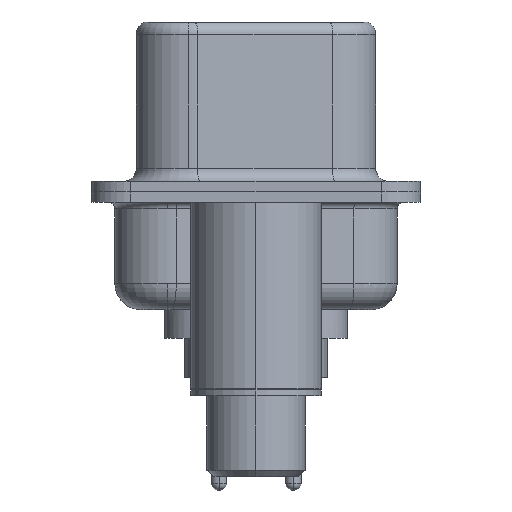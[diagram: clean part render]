
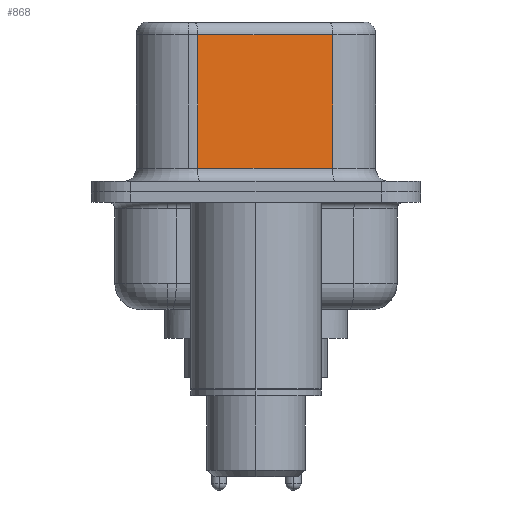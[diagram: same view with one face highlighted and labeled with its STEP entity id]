
A CAD part, left-side view. The second image highlights one B-rep face of the part: STEP entity #868.
In plain terms, the highlighted planar face has unit normal (-0.985, -0.174, 0).
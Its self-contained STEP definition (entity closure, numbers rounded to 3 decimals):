
#770 = ORIENTED_EDGE ( 'NONE', *, *, #19619, .T. ) ;
#868 = ADVANCED_FACE ( 'NONE', ( #7350 ), #15863, .F. ) ;
#1014 = VERTEX_POINT ( 'NONE', #7657 ) ;
#1169 = LINE ( 'NONE', #13580, #13796 ) ;
#1703 = CARTESIAN_POINT ( 'NONE',  ( 4.585, -2.927, 6.52 ) ) ;
#1913 = LINE ( 'NONE', #5136, #19495 ) ;
#3232 = LINE ( 'NONE', #15516, #7013 ) ;
#3485 = EDGE_CURVE ( 'NONE', #1014, #19299, #1169, .T. ) ;
#4028 = AXIS2_PLACEMENT_3D ( 'NONE', #1703, #16682, #13517 ) ;
#4125 = EDGE_LOOP ( 'NONE', ( #13863, #770, #20243, #10467 ) ) ;
#4358 = DIRECTION ( 'NONE',  ( 0., 0., -1. ) ) ;
#5078 = EDGE_CURVE ( 'NONE', #18880, #19299, #3232, .T. ) ;
#5136 = CARTESIAN_POINT ( 'NONE',  ( 4.585, -2.927, 6.02 ) ) ;
#6142 = CARTESIAN_POINT ( 'NONE',  ( 3.675, 2.233, 6.52 ) ) ;
#6674 = EDGE_CURVE ( 'NONE', #9554, #1014, #16602, .T. ) ;
#7013 = VECTOR ( 'NONE', #4358, 1000. ) ;
#7350 = FACE_OUTER_BOUND ( 'NONE', #4125, .T. ) ;
#7657 = CARTESIAN_POINT ( 'NONE',  ( 3.675, 2.233, 0.9 ) ) ;
#9115 = DIRECTION ( 'NONE',  ( 0.174, -0.985, 0. ) ) ;
#9554 = VERTEX_POINT ( 'NONE', #17928 ) ;
#10023 = DIRECTION ( 'NONE',  ( 0., 0., -1. ) ) ;
#10467 = ORIENTED_EDGE ( 'NONE', *, *, #3485, .T. ) ;
#13357 = DIRECTION ( 'NONE',  ( -0.174, 0.985, 0. ) ) ;
#13517 = DIRECTION ( 'NONE',  ( -0.174, 0.985, 0. ) ) ;
#13580 = CARTESIAN_POINT ( 'NONE',  ( 4.585, -2.927, 0.9 ) ) ;
#13796 = VECTOR ( 'NONE', #9115, 1000. ) ;
#13863 = ORIENTED_EDGE ( 'NONE', *, *, #5078, .F. ) ;
#15516 = CARTESIAN_POINT ( 'NONE',  ( 4.585, -2.927, 6.52 ) ) ;
#15863 = PLANE ( 'NONE',  #4028 ) ;
#16108 = VECTOR ( 'NONE', #10023, 1000. ) ;
#16602 = LINE ( 'NONE', #6142, #16108 ) ;
#16682 = DIRECTION ( 'NONE',  ( 0.985, 0.174, 0. ) ) ;
#16723 = CARTESIAN_POINT ( 'NONE',  ( 4.585, -2.927, 6.02 ) ) ;
#17928 = CARTESIAN_POINT ( 'NONE',  ( 3.675, 2.233, 6.02 ) ) ;
#18880 = VERTEX_POINT ( 'NONE', #16723 ) ;
#19299 = VERTEX_POINT ( 'NONE', #20959 ) ;
#19495 = VECTOR ( 'NONE', #13357, 1000. ) ;
#19619 = EDGE_CURVE ( 'NONE', #18880, #9554, #1913, .T. ) ;
#20243 = ORIENTED_EDGE ( 'NONE', *, *, #6674, .T. ) ;
#20959 = CARTESIAN_POINT ( 'NONE',  ( 4.585, -2.927, 0.9 ) ) ;
